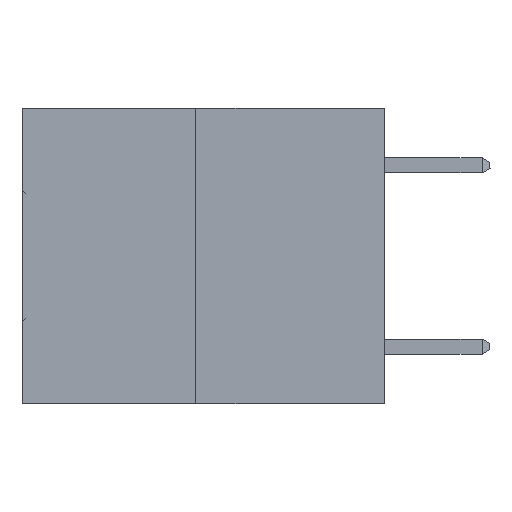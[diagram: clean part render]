
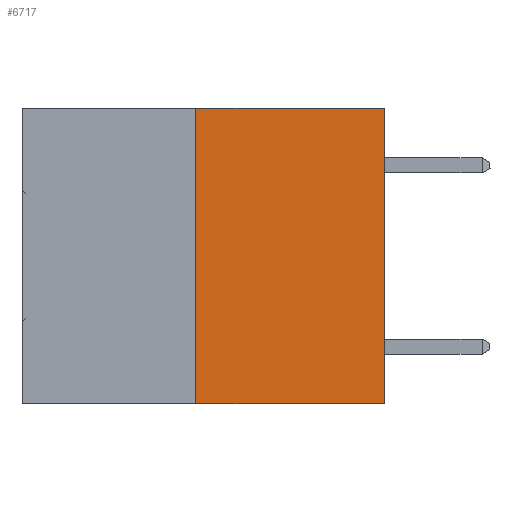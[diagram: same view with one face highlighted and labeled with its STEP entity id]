
A CAD part, left-side view. The second image highlights one B-rep face of the part: STEP entity #6717.
In plain terms, the highlighted planar face has unit normal (-1, 0, 0).
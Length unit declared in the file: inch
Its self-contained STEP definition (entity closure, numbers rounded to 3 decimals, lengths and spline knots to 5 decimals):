
#548 = LINE ( 'NONE', #4111, #29980 ) ;
#1136 = EDGE_CURVE ( 'NONE', #3461, #5349, #548, .T. ) ;
#3461 = VERTEX_POINT ( 'NONE', #37485 ) ;
#3709 = ORIENTED_EDGE ( 'NONE', *, *, #30149, .T. ) ;
#4111 = CARTESIAN_POINT ( 'NONE',  ( 0., 0.6, 0. ) ) ;
#4790 = ORIENTED_EDGE ( 'NONE', *, *, #29749, .T. ) ;
#5050 = DIRECTION ( 'NONE',  ( 0., 0., 1. ) ) ;
#5349 = VERTEX_POINT ( 'NONE', #23551 ) ;
#6091 = CARTESIAN_POINT ( 'NONE',  ( 0., 0., 0. ) ) ;
#6410 = EDGE_CURVE ( 'NONE', #23186, #3461, #22971, .T. ) ;
#6717 = ADVANCED_FACE ( 'NONE', ( #22933 ), #14612, .F. ) ;
#8582 = CARTESIAN_POINT ( 'NONE',  ( 0., 0.6, 0. ) ) ;
#9189 = CARTESIAN_POINT ( 'NONE',  ( 0., 0., -0.49 ) ) ;
#10511 = AXIS2_PLACEMENT_3D ( 'NONE', #8582, #32529, #20981 ) ;
#10646 = CARTESIAN_POINT ( 'NONE',  ( 0., 0.312, -0.49 ) ) ;
#10907 = VECTOR ( 'NONE', #5050, 39.37008 ) ;
#13198 = LINE ( 'NONE', #34828, #20048 ) ;
#14612 = PLANE ( 'NONE',  #10511 ) ;
#15130 = DIRECTION ( 'NONE',  ( 0., -1., 0. ) ) ;
#17659 = CARTESIAN_POINT ( 'NONE',  ( 0., 0.312, -0.49 ) ) ;
#18782 = DIRECTION ( 'NONE',  ( 0., -1., 0. ) ) ;
#19562 = LINE ( 'NONE', #6091, #10907 ) ;
#20048 = VECTOR ( 'NONE', #15130, 39.37008 ) ;
#20981 = DIRECTION ( 'NONE',  ( 0., 0., -1. ) ) ;
#22156 = EDGE_LOOP ( 'NONE', ( #30346, #4790, #3709, #31611 ) ) ;
#22933 = FACE_OUTER_BOUND ( 'NONE', #22156, .T. ) ;
#22971 = LINE ( 'NONE', #17659, #30906 ) ;
#23186 = VERTEX_POINT ( 'NONE', #10646 ) ;
#23342 = DIRECTION ( 'NONE',  ( 0., 0., 1. ) ) ;
#23551 = CARTESIAN_POINT ( 'NONE',  ( 0., 0., 0. ) ) ;
#29749 = EDGE_CURVE ( 'NONE', #23186, #32107, #13198, .T. ) ;
#29980 = VECTOR ( 'NONE', #18782, 39.37008 ) ;
#30149 = EDGE_CURVE ( 'NONE', #32107, #5349, #19562, .T. ) ;
#30346 = ORIENTED_EDGE ( 'NONE', *, *, #6410, .F. ) ;
#30906 = VECTOR ( 'NONE', #23342, 39.37008 ) ;
#31611 = ORIENTED_EDGE ( 'NONE', *, *, #1136, .F. ) ;
#32107 = VERTEX_POINT ( 'NONE', #9189 ) ;
#32529 = DIRECTION ( 'NONE',  ( 1., 0., 0. ) ) ;
#34828 = CARTESIAN_POINT ( 'NONE',  ( 0., 0.6, -0.49 ) ) ;
#37485 = CARTESIAN_POINT ( 'NONE',  ( 0., 0.312, 0. ) ) ;
